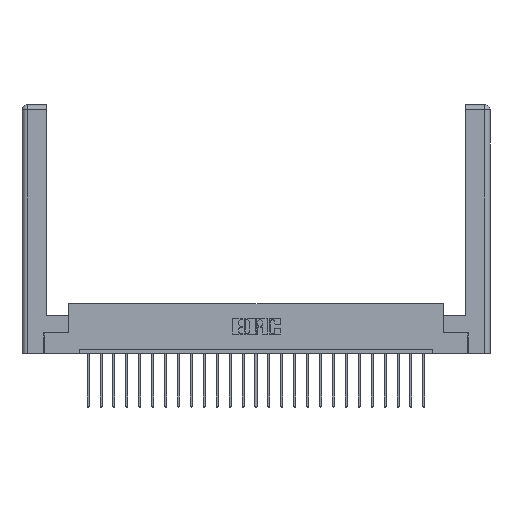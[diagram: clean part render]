
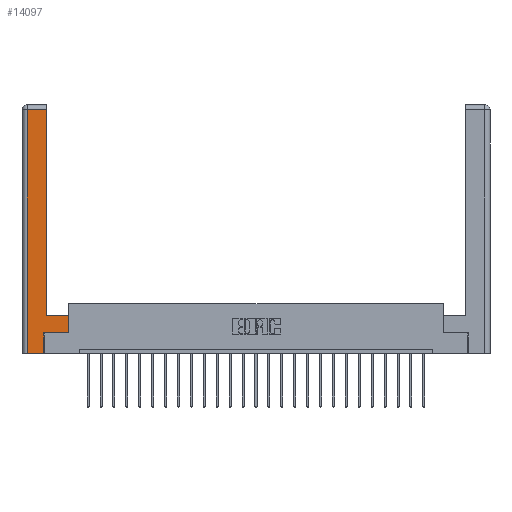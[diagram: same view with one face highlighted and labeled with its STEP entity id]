
A CAD part, top view. The second image highlights one B-rep face of the part: STEP entity #14097.
In plain terms, the highlighted planar face has unit normal (0, 0, 1).
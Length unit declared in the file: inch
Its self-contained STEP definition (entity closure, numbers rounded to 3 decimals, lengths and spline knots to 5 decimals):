
#79 = DIRECTION ( 'NONE',  ( 1., 0., 0. ) ) ;
#409 = LINE ( 'NONE', #4431, #18570 ) ;
#961 = DIRECTION ( 'NONE',  ( 0., 1., 0. ) ) ;
#1329 = LINE ( 'NONE', #19816, #7004 ) ;
#1424 = CARTESIAN_POINT ( 'NONE',  ( 0.0615, 2.94, 0. ) ) ;
#2049 = DIRECTION ( 'NONE',  ( 0., 1., 0. ) ) ;
#2257 = CARTESIAN_POINT ( 'NONE',  ( 0.265, 0.245, 0. ) ) ;
#2538 = VERTEX_POINT ( 'NONE', #9820 ) ;
#2930 = ORIENTED_EDGE ( 'NONE', *, *, #4980, .T. ) ;
#3016 = EDGE_CURVE ( 'NONE', #9047, #11039, #14663, .T. ) ;
#3347 = VECTOR ( 'NONE', #79, 39.37008 ) ;
#3630 = EDGE_LOOP ( 'NONE', ( #23845, #12612, #8917, #4702, #15942, #20625, #2930, #9236 ) ) ;
#3815 = LINE ( 'NONE', #6121, #3347 ) ;
#4431 = CARTESIAN_POINT ( 'NONE',  ( 0.0615, 0., 0. ) ) ;
#4702 = ORIENTED_EDGE ( 'NONE', *, *, #23336, .T. ) ;
#4980 = EDGE_CURVE ( 'NONE', #20222, #15867, #5904, .T. ) ;
#5786 = CARTESIAN_POINT ( 'NONE',  ( 0.565, 0.45, 0. ) ) ;
#5823 = DIRECTION ( 'NONE',  ( 0., 0., -1. ) ) ;
#5853 = EDGE_CURVE ( 'NONE', #17536, #9047, #9782, .T. ) ;
#5904 = LINE ( 'NONE', #15578, #9473 ) ;
#6121 = CARTESIAN_POINT ( 'NONE',  ( 0.565, 0.245, 0. ) ) ;
#6148 = PLANE ( 'NONE',  #9331 ) ;
#7004 = VECTOR ( 'NONE', #8407, 39.37008 ) ;
#7257 = EDGE_CURVE ( 'NONE', #2538, #18489, #12385, .T. ) ;
#7444 = VECTOR ( 'NONE', #19034, 39.37008 ) ;
#7741 = EDGE_CURVE ( 'NONE', #15867, #17536, #1329, .T. ) ;
#8407 = DIRECTION ( 'NONE',  ( -1., 0., 0. ) ) ;
#8917 = ORIENTED_EDGE ( 'NONE', *, *, #11824, .T. ) ;
#9047 = VERTEX_POINT ( 'NONE', #17440 ) ;
#9236 = ORIENTED_EDGE ( 'NONE', *, *, #7741, .T. ) ;
#9331 = AXIS2_PLACEMENT_3D ( 'NONE', #13818, #5823, #17348 ) ;
#9394 = VECTOR ( 'NONE', #2049, 39.37008 ) ;
#9457 = CARTESIAN_POINT ( 'NONE',  ( 0.265, 0., 0. ) ) ;
#9473 = VECTOR ( 'NONE', #21063, 39.37008 ) ;
#9782 = LINE ( 'NONE', #20103, #15139 ) ;
#9820 = CARTESIAN_POINT ( 'NONE',  ( 0.265, 0., 0. ) ) ;
#10347 = VERTEX_POINT ( 'NONE', #16561 ) ;
#11039 = VERTEX_POINT ( 'NONE', #1424 ) ;
#11057 = VECTOR ( 'NONE', #22135, 39.37008 ) ;
#11824 = EDGE_CURVE ( 'NONE', #11039, #10347, #409, .T. ) ;
#12385 = LINE ( 'NONE', #17242, #9394 ) ;
#12612 = ORIENTED_EDGE ( 'NONE', *, *, #3016, .T. ) ;
#13818 = CARTESIAN_POINT ( 'NONE',  ( 0., 0., 0. ) ) ;
#14097 = ADVANCED_FACE ( 'NONE', ( #19345 ), #6148, .F. ) ;
#14300 = CARTESIAN_POINT ( 'NONE',  ( 0.0615, 2.94, 0. ) ) ;
#14663 = LINE ( 'NONE', #14300, #11057 ) ;
#15139 = VECTOR ( 'NONE', #961, 39.37008 ) ;
#15578 = CARTESIAN_POINT ( 'NONE',  ( 0.565, 0.45, 0. ) ) ;
#15867 = VERTEX_POINT ( 'NONE', #5786 ) ;
#15942 = ORIENTED_EDGE ( 'NONE', *, *, #7257, .T. ) ;
#16561 = CARTESIAN_POINT ( 'NONE',  ( 0.0615, 0., 0. ) ) ;
#17242 = CARTESIAN_POINT ( 'NONE',  ( 0.265, 0.245, 0. ) ) ;
#17348 = DIRECTION ( 'NONE',  ( -1., 0., 0. ) ) ;
#17440 = CARTESIAN_POINT ( 'NONE',  ( 0.295, 2.94, 0. ) ) ;
#17536 = VERTEX_POINT ( 'NONE', #18660 ) ;
#18223 = LINE ( 'NONE', #9457, #7444 ) ;
#18489 = VERTEX_POINT ( 'NONE', #2257 ) ;
#18570 = VECTOR ( 'NONE', #23434, 39.37008 ) ;
#18660 = CARTESIAN_POINT ( 'NONE',  ( 0.295, 0.45, 0. ) ) ;
#19034 = DIRECTION ( 'NONE',  ( 1., 0., 0. ) ) ;
#19345 = FACE_OUTER_BOUND ( 'NONE', #3630, .T. ) ;
#19816 = CARTESIAN_POINT ( 'NONE',  ( 0.295, 0.45, 0. ) ) ;
#20103 = CARTESIAN_POINT ( 'NONE',  ( 0.295, 3., 0. ) ) ;
#20222 = VERTEX_POINT ( 'NONE', #24476 ) ;
#20625 = ORIENTED_EDGE ( 'NONE', *, *, #21588, .T. ) ;
#21063 = DIRECTION ( 'NONE',  ( 0., 1., 0. ) ) ;
#21588 = EDGE_CURVE ( 'NONE', #18489, #20222, #3815, .T. ) ;
#22135 = DIRECTION ( 'NONE',  ( -1., 0., 0. ) ) ;
#23336 = EDGE_CURVE ( 'NONE', #10347, #2538, #18223, .T. ) ;
#23434 = DIRECTION ( 'NONE',  ( 0., -1., 0. ) ) ;
#23845 = ORIENTED_EDGE ( 'NONE', *, *, #5853, .T. ) ;
#24476 = CARTESIAN_POINT ( 'NONE',  ( 0.565, 0.245, 0. ) ) ;
